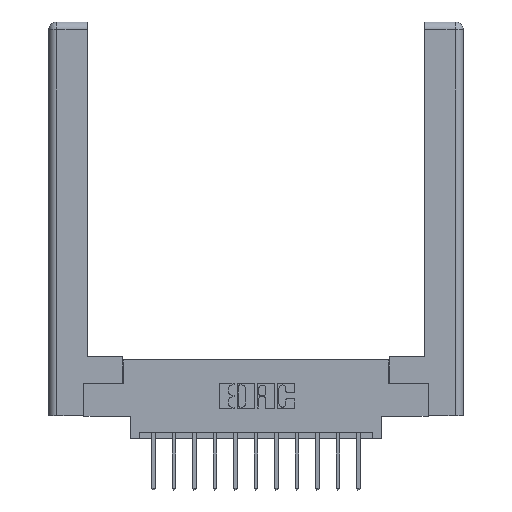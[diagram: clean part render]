
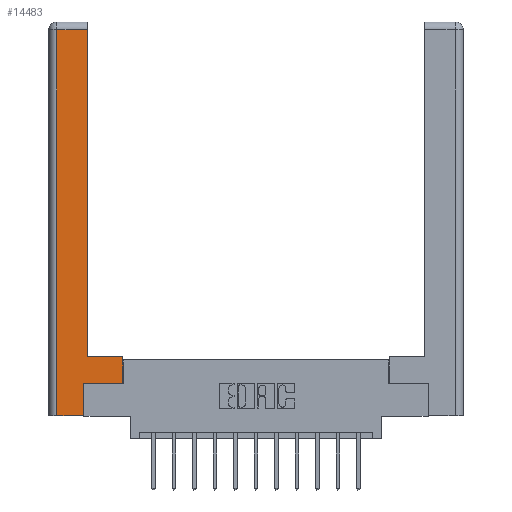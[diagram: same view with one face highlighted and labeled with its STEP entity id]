
A CAD part, top view. The second image highlights one B-rep face of the part: STEP entity #14483.
In plain terms, the highlighted planar face has unit normal (0, 0, 1).
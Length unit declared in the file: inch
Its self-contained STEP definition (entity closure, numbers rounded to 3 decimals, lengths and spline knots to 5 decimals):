
#50 = EDGE_LOOP ( 'NONE', ( #3933, #6453, #7481, #11196, #14428, #9345, #12422, #12713 ) ) ;
#287 = DIRECTION ( 'NONE',  ( 0., 0., -1. ) ) ;
#364 = VECTOR ( 'NONE', #11406, 39.37008 ) ;
#918 = CARTESIAN_POINT ( 'NONE',  ( 0.265, 0., 0. ) ) ;
#1071 = CARTESIAN_POINT ( 'NONE',  ( 0.565, 0.245, 0. ) ) ;
#1099 = CARTESIAN_POINT ( 'NONE',  ( 0.295, 2.94, 0. ) ) ;
#1773 = LINE ( 'NONE', #5709, #7143 ) ;
#2212 = VERTEX_POINT ( 'NONE', #1071 ) ;
#2361 = CARTESIAN_POINT ( 'NONE',  ( 0.0615, 2.94, 0. ) ) ;
#2544 = CARTESIAN_POINT ( 'NONE',  ( 0.565, 0.245, 0. ) ) ;
#2813 = CARTESIAN_POINT ( 'NONE',  ( 0.295, 0.45, 0. ) ) ;
#2849 = EDGE_CURVE ( 'NONE', #9810, #3230, #7520, .T. ) ;
#3230 = VERTEX_POINT ( 'NONE', #9607 ) ;
#3436 = DIRECTION ( 'NONE',  ( 0., 1., 0. ) ) ;
#3441 = FACE_OUTER_BOUND ( 'NONE', #50, .T. ) ;
#3446 = VERTEX_POINT ( 'NONE', #1099 ) ;
#3533 = EDGE_CURVE ( 'NONE', #3230, #12723, #1773, .T. ) ;
#3582 = CARTESIAN_POINT ( 'NONE',  ( 0.295, 3., 0. ) ) ;
#3633 = CARTESIAN_POINT ( 'NONE',  ( 0.265, 0.245, 0. ) ) ;
#3818 = DIRECTION ( 'NONE',  ( -1., 0., 0. ) ) ;
#3825 = VECTOR ( 'NONE', #3436, 39.37008 ) ;
#3920 = CARTESIAN_POINT ( 'NONE',  ( 0., 0., 0. ) ) ;
#3933 = ORIENTED_EDGE ( 'NONE', *, *, #5520, .T. ) ;
#4323 = VECTOR ( 'NONE', #10886, 39.37008 ) ;
#4508 = LINE ( 'NONE', #11955, #4323 ) ;
#4804 = DIRECTION ( 'NONE',  ( 1., 0., 0. ) ) ;
#5179 = DIRECTION ( 'NONE',  ( 0., 1., 0. ) ) ;
#5362 = VERTEX_POINT ( 'NONE', #2361 ) ;
#5450 = VECTOR ( 'NONE', #6778, 39.37008 ) ;
#5520 = EDGE_CURVE ( 'NONE', #8983, #3446, #8252, .T. ) ;
#5709 = CARTESIAN_POINT ( 'NONE',  ( 0.265, 0.245, 0. ) ) ;
#5763 = LINE ( 'NONE', #10230, #364 ) ;
#6200 = LINE ( 'NONE', #6831, #5450 ) ;
#6337 = AXIS2_PLACEMENT_3D ( 'NONE', #3920, #287, #3818 ) ;
#6449 = CARTESIAN_POINT ( 'NONE',  ( 0.565, 0.45, 0. ) ) ;
#6453 = ORIENTED_EDGE ( 'NONE', *, *, #9264, .T. ) ;
#6778 = DIRECTION ( 'NONE',  ( 0., -1., 0. ) ) ;
#6831 = CARTESIAN_POINT ( 'NONE',  ( 0.0615, 0., 0. ) ) ;
#7143 = VECTOR ( 'NONE', #12715, 39.37008 ) ;
#7211 = VERTEX_POINT ( 'NONE', #8039 ) ;
#7481 = ORIENTED_EDGE ( 'NONE', *, *, #11861, .T. ) ;
#7520 = LINE ( 'NONE', #918, #15312 ) ;
#8039 = CARTESIAN_POINT ( 'NONE',  ( 0.565, 0.45, 0. ) ) ;
#8143 = DIRECTION ( 'NONE',  ( 1., 0., 0. ) ) ;
#8252 = LINE ( 'NONE', #3582, #3825 ) ;
#8983 = VERTEX_POINT ( 'NONE', #2813 ) ;
#9264 = EDGE_CURVE ( 'NONE', #3446, #5362, #5763, .T. ) ;
#9345 = ORIENTED_EDGE ( 'NONE', *, *, #10879, .T. ) ;
#9607 = CARTESIAN_POINT ( 'NONE',  ( 0.265, 0., 0. ) ) ;
#9810 = VERTEX_POINT ( 'NONE', #12583 ) ;
#10103 = VECTOR ( 'NONE', #4804, 39.37008 ) ;
#10230 = CARTESIAN_POINT ( 'NONE',  ( 0.0615, 2.94, 0. ) ) ;
#10322 = VECTOR ( 'NONE', #5179, 39.37008 ) ;
#10879 = EDGE_CURVE ( 'NONE', #12723, #2212, #14792, .T. ) ;
#10886 = DIRECTION ( 'NONE',  ( -1., 0., 0. ) ) ;
#11196 = ORIENTED_EDGE ( 'NONE', *, *, #2849, .T. ) ;
#11406 = DIRECTION ( 'NONE',  ( -1., 0., 0. ) ) ;
#11861 = EDGE_CURVE ( 'NONE', #5362, #9810, #6200, .T. ) ;
#11955 = CARTESIAN_POINT ( 'NONE',  ( 0.295, 0.45, 0. ) ) ;
#12422 = ORIENTED_EDGE ( 'NONE', *, *, #15196, .T. ) ;
#12583 = CARTESIAN_POINT ( 'NONE',  ( 0.0615, 0., 0. ) ) ;
#12711 = EDGE_CURVE ( 'NONE', #7211, #8983, #4508, .T. ) ;
#12713 = ORIENTED_EDGE ( 'NONE', *, *, #12711, .T. ) ;
#12715 = DIRECTION ( 'NONE',  ( 0., 1., 0. ) ) ;
#12723 = VERTEX_POINT ( 'NONE', #3633 ) ;
#14428 = ORIENTED_EDGE ( 'NONE', *, *, #3533, .T. ) ;
#14430 = PLANE ( 'NONE',  #6337 ) ;
#14437 = LINE ( 'NONE', #6449, #10322 ) ;
#14483 = ADVANCED_FACE ( 'NONE', ( #3441 ), #14430, .F. ) ;
#14792 = LINE ( 'NONE', #2544, #10103 ) ;
#15196 = EDGE_CURVE ( 'NONE', #2212, #7211, #14437, .T. ) ;
#15312 = VECTOR ( 'NONE', #8143, 39.37008 ) ;
